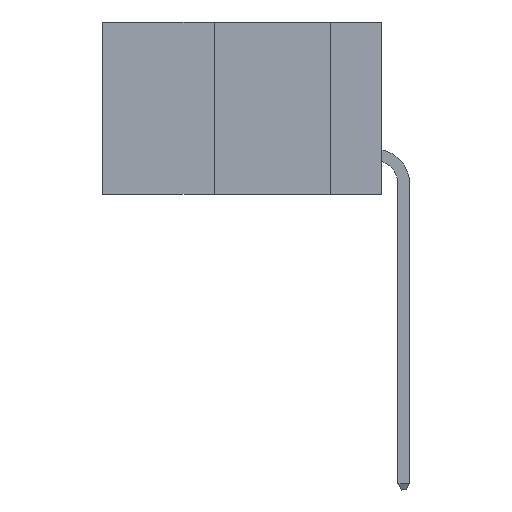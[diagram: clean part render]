
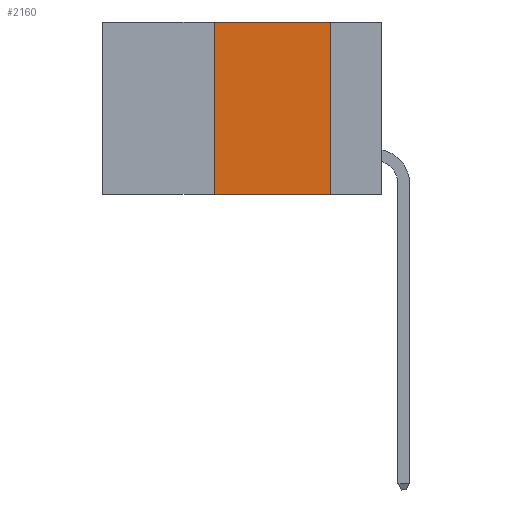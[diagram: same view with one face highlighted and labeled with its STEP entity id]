
A CAD part, left-side view. The second image highlights one B-rep face of the part: STEP entity #2160.
In plain terms, the highlighted planar face has unit normal (-1, 0, 0).
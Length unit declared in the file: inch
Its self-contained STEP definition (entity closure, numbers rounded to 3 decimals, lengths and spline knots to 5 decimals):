
#566 = EDGE_CURVE ( 'NONE', #689, #13531, #13881, .T. ) ;
#689 = VERTEX_POINT ( 'NONE', #2408 ) ;
#1728 = EDGE_CURVE ( 'NONE', #689, #12829, #9780, .T. ) ;
#2108 = CARTESIAN_POINT ( 'NONE',  ( 0., 0.11, -0.37 ) ) ;
#2160 = ADVANCED_FACE ( 'NONE', ( #6441 ), #5249, .F. ) ;
#2216 = VECTOR ( 'NONE', #3922, 39.37008 ) ;
#2408 = CARTESIAN_POINT ( 'NONE',  ( 0., 0.36, -0.37 ) ) ;
#2799 = CARTESIAN_POINT ( 'NONE',  ( 0., 0.36, 0. ) ) ;
#3058 = ORIENTED_EDGE ( 'NONE', *, *, #566, .T. ) ;
#3759 = AXIS2_PLACEMENT_3D ( 'NONE', #8545, #5205, #6433 ) ;
#3922 = DIRECTION ( 'NONE',  ( 0., 0., -1. ) ) ;
#4151 = EDGE_CURVE ( 'NONE', #12829, #7081, #9727, .T. ) ;
#4887 = ORIENTED_EDGE ( 'NONE', *, *, #1728, .F. ) ;
#5205 = DIRECTION ( 'NONE',  ( 1., 0., 0. ) ) ;
#5249 = PLANE ( 'NONE',  #3759 ) ;
#5669 = ORIENTED_EDGE ( 'NONE', *, *, #4151, .F. ) ;
#6145 = VECTOR ( 'NONE', #7647, 39.37008 ) ;
#6207 = EDGE_LOOP ( 'NONE', ( #13470, #5669, #4887, #3058 ) ) ;
#6433 = DIRECTION ( 'NONE',  ( 0., 0., -1. ) ) ;
#6441 = FACE_OUTER_BOUND ( 'NONE', #6207, .T. ) ;
#6604 = DIRECTION ( 'NONE',  ( 0., -1., 0. ) ) ;
#7081 = VERTEX_POINT ( 'NONE', #9657 ) ;
#7119 = DIRECTION ( 'NONE',  ( 0., 0., 1. ) ) ;
#7647 = DIRECTION ( 'NONE',  ( 0., -1., 0. ) ) ;
#8545 = CARTESIAN_POINT ( 'NONE',  ( 0., 0.6, 0. ) ) ;
#9657 = CARTESIAN_POINT ( 'NONE',  ( 0., 0.11, 0. ) ) ;
#9727 = LINE ( 'NONE', #14360, #12893 ) ;
#9780 = LINE ( 'NONE', #2799, #14176 ) ;
#10776 = CARTESIAN_POINT ( 'NONE',  ( 0., 0.36, 0. ) ) ;
#11168 = CARTESIAN_POINT ( 'NONE',  ( 0., 0.6, -0.37 ) ) ;
#11352 = EDGE_CURVE ( 'NONE', #7081, #13531, #14130, .T. ) ;
#12829 = VERTEX_POINT ( 'NONE', #10776 ) ;
#12893 = VECTOR ( 'NONE', #6604, 39.37008 ) ;
#12976 = CARTESIAN_POINT ( 'NONE',  ( 0., 0.11, 0. ) ) ;
#13470 = ORIENTED_EDGE ( 'NONE', *, *, #11352, .F. ) ;
#13531 = VERTEX_POINT ( 'NONE', #2108 ) ;
#13881 = LINE ( 'NONE', #11168, #6145 ) ;
#14130 = LINE ( 'NONE', #12976, #2216 ) ;
#14176 = VECTOR ( 'NONE', #7119, 39.37008 ) ;
#14360 = CARTESIAN_POINT ( 'NONE',  ( 0., 0.6, 0. ) ) ;
